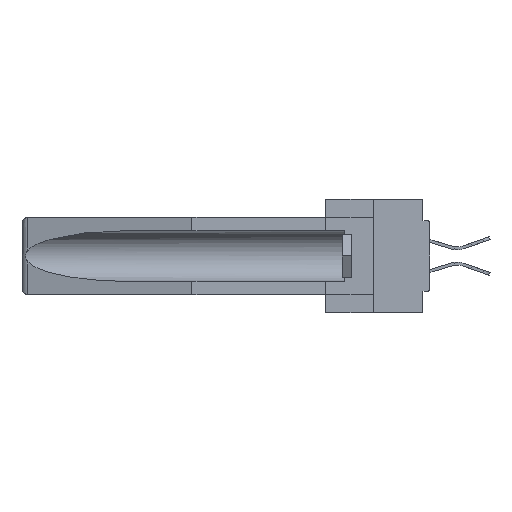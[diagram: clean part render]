
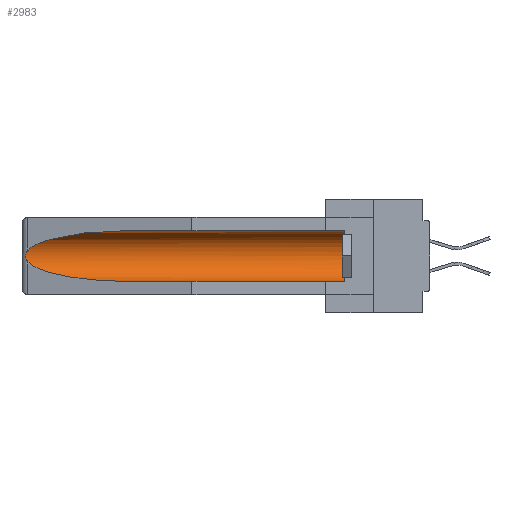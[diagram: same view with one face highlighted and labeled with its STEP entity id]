
A CAD part, left-side view. The second image highlights one B-rep face of the part: STEP entity #2983.
In plain terms, the highlighted cylindrical face has radius 2.857 mm (diameter 5.715 mm), a partial arc.
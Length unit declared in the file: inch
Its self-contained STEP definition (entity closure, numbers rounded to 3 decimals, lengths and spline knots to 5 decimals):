
#2318 = CARTESIAN_POINT ( 'NONE',  ( 0.26537, 1.52718, -0.14972 ) ) ;
#2983 = ADVANCED_FACE ( 'NONE', ( #21801 ), #12384, .F. ) ;
#4371 = CARTESIAN_POINT ( 'NONE',  ( 0.26597, 1.52961, -0.15275 ) ) ;
#4393 = VECTOR ( 'NONE', #23605, 39.37008 ) ;
#4501 = CARTESIAN_POINT ( 'NONE',  ( 0.26537, 1.52718, -0.19328 ) ) ;
#6913 = EDGE_CURVE ( 'NONE', #8081, #25515, #12280, .T. ) ;
#7252 = CARTESIAN_POINT ( 'NONE',  ( 0.25451, 1.48313, -0.09465 ) ) ;
#7396 = VERTEX_POINT ( 'NONE', #14329 ) ;
#7579 = ORIENTED_EDGE ( 'NONE', *, *, #27893, .F. ) ;
#7615 = CARTESIAN_POINT ( 'NONE',  ( 0.2673, 1.5327, -0.16383 ) ) ;
#8081 = VERTEX_POINT ( 'NONE', #23200 ) ;
#10123 = CARTESIAN_POINT ( 'NONE',  ( 0.2675, 1.53308, -0.16763 ) ) ;
#11011 = CARTESIAN_POINT ( 'NONE',  ( 0.25451, 1.48313, -0.24835 ) ) ;
#12280 =( BOUNDED_CURVE ( )  B_SPLINE_CURVE ( 3, ( #28983, #11011, #23226, #37950 ),
 .UNSPECIFIED., .F., .F. ) 
 B_SPLINE_CURVE_WITH_KNOTS ( ( 4, 4 ),
 ( 0.1948, 1.5708 ),
 .UNSPECIFIED. ) 
 CURVE ( )  GEOMETRIC_REPRESENTATION_ITEM ( )  RATIONAL_B_SPLINE_CURVE ( ( 1., 0.848, 0.848, 1. ) ) 
 REPRESENTATION_ITEM ( '' )  );
#12384 = CYLINDRICAL_SURFACE ( 'NONE', #35444, 0.1125 ) ;
#12930 = ORIENTED_EDGE ( 'NONE', *, *, #19047, .T. ) ;
#13244 = CARTESIAN_POINT ( 'NONE',  ( 0.26655, 1.53094, -0.18657 ) ) ;
#14054 = EDGE_CURVE ( 'NONE', #35169, #36956, #14634, .T. ) ;
#14169 = DIRECTION ( 'NONE',  ( 0., 0., 1. ) ) ;
#14329 = CARTESIAN_POINT ( 'NONE',  ( 0.155, 0.126, -0.284 ) ) ;
#14623 = CARTESIAN_POINT ( 'NONE',  ( 0.155, -0.30754, -0.059 ) ) ;
#14634 = LINE ( 'NONE', #14623, #4393 ) ;
#14960 = DIRECTION ( 'NONE',  ( 0., -1., 0. ) ) ;
#15707 = ORIENTED_EDGE ( 'NONE', *, *, #6913, .T. ) ;
#18617 = CIRCLE ( 'NONE', #20524, 0.1125 ) ;
#19046 = CARTESIAN_POINT ( 'NONE',  ( 0.26597, 1.5296, -0.19026 ) ) ;
#19047 = EDGE_CURVE ( 'NONE', #20596, #8081, #35650, .T. ) ;
#19510 = CARTESIAN_POINT ( 'NONE',  ( 0.155, -0.30754, -0.284 ) ) ;
#20166 = CARTESIAN_POINT ( 'NONE',  ( 0.155, 1.07973, -0.284 ) ) ;
#20524 = AXIS2_PLACEMENT_3D ( 'NONE', #35661, #14960, #38813 ) ;
#20596 = VERTEX_POINT ( 'NONE', #2318 ) ;
#21542 = EDGE_LOOP ( 'NONE', ( #27050, #12930, #15707, #7579, #33021, #30187 ) ) ;
#21801 = FACE_OUTER_BOUND ( 'NONE', #21542, .T. ) ;
#22575 = VECTOR ( 'NONE', #34627, 39.37008 ) ;
#22970 = CARTESIAN_POINT ( 'NONE',  ( 0.26537, 1.52718, -0.14972 ) ) ;
#23200 = CARTESIAN_POINT ( 'NONE',  ( 0.26537, 1.52718, -0.19328 ) ) ;
#23226 = CARTESIAN_POINT ( 'NONE',  ( 0.21114, 1.30732, -0.284 ) ) ;
#23605 = DIRECTION ( 'NONE',  ( 0., 1., 0. ) ) ;
#24638 = CARTESIAN_POINT ( 'NONE',  ( 0.155, 0.126, -0.059 ) ) ;
#25228 = CARTESIAN_POINT ( 'NONE',  ( 0.2673, 1.53269, -0.17917 ) ) ;
#25515 = VERTEX_POINT ( 'NONE', #20166 ) ;
#26144 = CARTESIAN_POINT ( 'NONE',  ( 0.155, -0.30754, -0.1715 ) ) ;
#27050 = ORIENTED_EDGE ( 'NONE', *, *, #31103, .T. ) ;
#27440 =( BOUNDED_CURVE ( )  B_SPLINE_CURVE ( 3, ( #34574, #37200, #7252, #22970 ),
 .UNSPECIFIED., .F., .F. ) 
 B_SPLINE_CURVE_WITH_KNOTS ( ( 4, 4 ),
 ( 4.71239, 6.08839 ),
 .UNSPECIFIED. ) 
 CURVE ( )  GEOMETRIC_REPRESENTATION_ITEM ( )  RATIONAL_B_SPLINE_CURVE ( ( 1., 0.848, 0.848, 1. ) ) 
 REPRESENTATION_ITEM ( '' )  );
#27893 = EDGE_CURVE ( 'NONE', #7396, #25515, #38961, .T. ) ;
#28239 = CARTESIAN_POINT ( 'NONE',  ( 0.26654, 1.53092, -0.15636 ) ) ;
#28983 = CARTESIAN_POINT ( 'NONE',  ( 0.26537, 1.52718, -0.19328 ) ) ;
#29020 = DIRECTION ( 'NONE',  ( 0., 1., 0. ) ) ;
#30187 = ORIENTED_EDGE ( 'NONE', *, *, #14054, .T. ) ;
#31103 = EDGE_CURVE ( 'NONE', #36956, #20596, #27440, .T. ) ;
#31239 = CARTESIAN_POINT ( 'NONE',  ( 0.2675, 1.53308, -0.17534 ) ) ;
#32614 = CARTESIAN_POINT ( 'NONE',  ( 0.155, 1.07973, -0.059 ) ) ;
#33021 = ORIENTED_EDGE ( 'NONE', *, *, #35381, .T. ) ;
#34574 = CARTESIAN_POINT ( 'NONE',  ( 0.155, 1.07973, -0.059 ) ) ;
#34627 = DIRECTION ( 'NONE',  ( 0., 1., 0. ) ) ;
#35169 = VERTEX_POINT ( 'NONE', #24638 ) ;
#35381 = EDGE_CURVE ( 'NONE', #7396, #35169, #18617, .T. ) ;
#35444 = AXIS2_PLACEMENT_3D ( 'NONE', #26144, #29020, #14169 ) ;
#35650 = B_SPLINE_CURVE_WITH_KNOTS ( 'NONE', 3,
 ( #37448, #4371, #28239, #7615, #10123, #31239, #25228, #13244, #19046, #4501 ),
 .UNSPECIFIED., .F., .F.,
 ( 4, 2, 2, 2, 4 ),
 ( 0., 0.00029, 0.00058, 0.00087, 0.00117 ),
 .UNSPECIFIED. ) ;
#35661 = CARTESIAN_POINT ( 'NONE',  ( 0.155, 0.126, -0.1715 ) ) ;
#36956 = VERTEX_POINT ( 'NONE', #32614 ) ;
#37200 = CARTESIAN_POINT ( 'NONE',  ( 0.21114, 1.30732, -0.059 ) ) ;
#37448 = CARTESIAN_POINT ( 'NONE',  ( 0.26537, 1.52718, -0.14972 ) ) ;
#37950 = CARTESIAN_POINT ( 'NONE',  ( 0.155, 1.07973, -0.284 ) ) ;
#38813 = DIRECTION ( 'NONE',  ( 0., 0., 1. ) ) ;
#38961 = LINE ( 'NONE', #19510, #22575 ) ;
